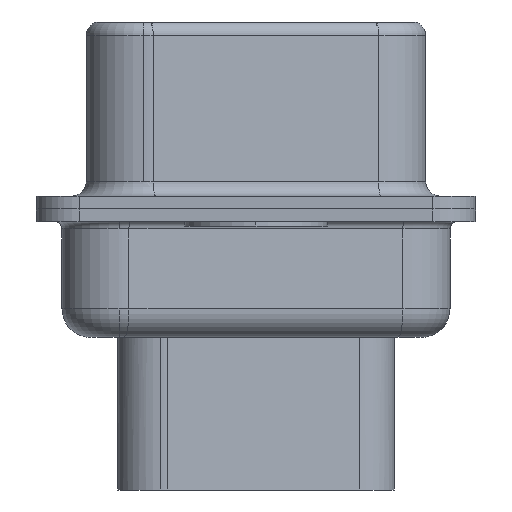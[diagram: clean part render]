
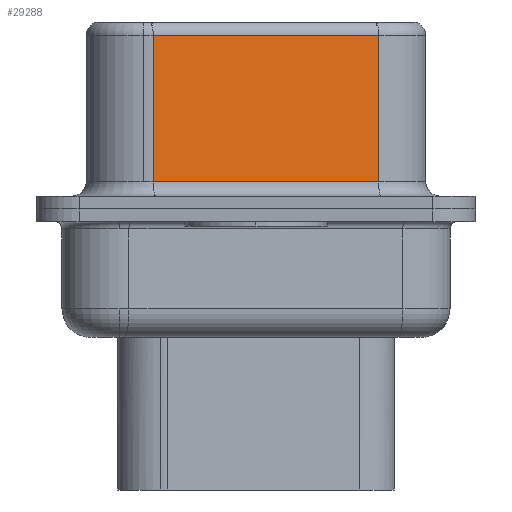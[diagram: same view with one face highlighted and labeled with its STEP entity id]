
A CAD part, left-side view. The second image highlights one B-rep face of the part: STEP entity #29288.
In plain terms, the highlighted planar face has unit normal (-0.985, -0.174, 0).
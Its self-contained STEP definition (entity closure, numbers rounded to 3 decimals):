
#185 = PLANE ( 'NONE',  #6867 ) ;
#1629 = CARTESIAN_POINT ( 'NONE',  ( 5.128, -4.297, 6.07 ) ) ;
#2840 = EDGE_LOOP ( 'NONE', ( #11690, #12910, #22543, #26228 ) ) ;
#3024 = CARTESIAN_POINT ( 'NONE',  ( 3.735, 3.603, 0.95 ) ) ;
#5076 = DIRECTION ( 'NONE',  ( -0.174, 0.985, 0. ) ) ;
#5505 = CARTESIAN_POINT ( 'NONE',  ( 5.128, -4.297, 0.95 ) ) ;
#6867 = AXIS2_PLACEMENT_3D ( 'NONE', #23328, #23784, #7575 ) ;
#7575 = DIRECTION ( 'NONE',  ( -0.174, 0.985, 0. ) ) ;
#7780 = LINE ( 'NONE', #23986, #21043 ) ;
#8133 = EDGE_CURVE ( 'NONE', #20070, #17003, #7780, .T. ) ;
#11690 = ORIENTED_EDGE ( 'NONE', *, *, #8133, .F. ) ;
#11862 = DIRECTION ( 'NONE',  ( 0.174, -0.985, 0. ) ) ;
#11945 = VERTEX_POINT ( 'NONE', #25894 ) ;
#11978 = VECTOR ( 'NONE', #22036, 1000. ) ;
#12167 = LINE ( 'NONE', #5505, #20889 ) ;
#12910 = ORIENTED_EDGE ( 'NONE', *, *, #28392, .T. ) ;
#14778 = LINE ( 'NONE', #28387, #28105 ) ;
#16721 = DIRECTION ( 'NONE',  ( 0., 0., -1. ) ) ;
#16886 = CARTESIAN_POINT ( 'NONE',  ( 3.735, 3.603, 6.57 ) ) ;
#17003 = VERTEX_POINT ( 'NONE', #24509 ) ;
#19101 = FACE_OUTER_BOUND ( 'NONE', #2840, .T. ) ;
#19315 = LINE ( 'NONE', #16886, #11978 ) ;
#19468 = VERTEX_POINT ( 'NONE', #3024 ) ;
#20070 = VERTEX_POINT ( 'NONE', #1629 ) ;
#20889 = VECTOR ( 'NONE', #11862, 1000. ) ;
#21043 = VECTOR ( 'NONE', #16721, 1000. ) ;
#22036 = DIRECTION ( 'NONE',  ( 0., 0., -1. ) ) ;
#22543 = ORIENTED_EDGE ( 'NONE', *, *, #23988, .T. ) ;
#23328 = CARTESIAN_POINT ( 'NONE',  ( 5.128, -4.297, 6.57 ) ) ;
#23784 = DIRECTION ( 'NONE',  ( 0.985, 0.174, 0. ) ) ;
#23986 = CARTESIAN_POINT ( 'NONE',  ( 5.128, -4.297, 6.57 ) ) ;
#23988 = EDGE_CURVE ( 'NONE', #11945, #19468, #19315, .T. ) ;
#24509 = CARTESIAN_POINT ( 'NONE',  ( 5.128, -4.297, 0.95 ) ) ;
#25894 = CARTESIAN_POINT ( 'NONE',  ( 3.735, 3.603, 6.07 ) ) ;
#26228 = ORIENTED_EDGE ( 'NONE', *, *, #28815, .T. ) ;
#28105 = VECTOR ( 'NONE', #5076, 1000. ) ;
#28387 = CARTESIAN_POINT ( 'NONE',  ( 5.128, -4.297, 6.07 ) ) ;
#28392 = EDGE_CURVE ( 'NONE', #20070, #11945, #14778, .T. ) ;
#28815 = EDGE_CURVE ( 'NONE', #19468, #17003, #12167, .T. ) ;
#29288 = ADVANCED_FACE ( 'NONE', ( #19101 ), #185, .F. ) ;
